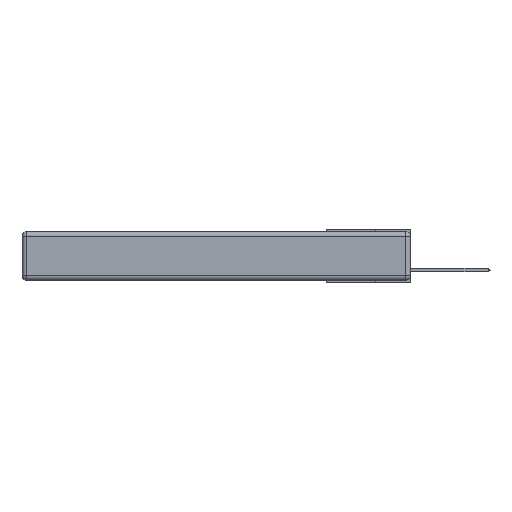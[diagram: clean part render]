
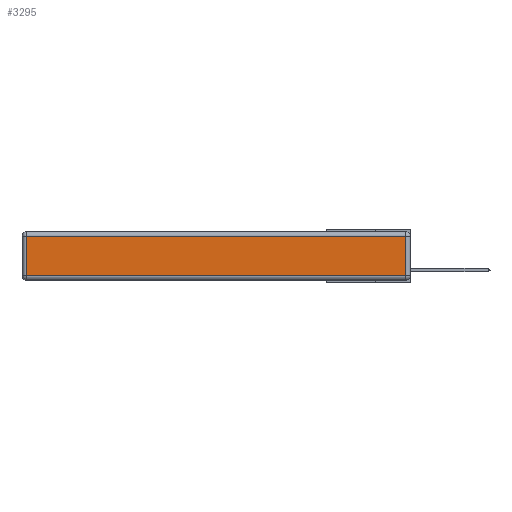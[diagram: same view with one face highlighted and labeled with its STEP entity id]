
A CAD part, left-side view. The second image highlights one B-rep face of the part: STEP entity #3295.
In plain terms, the highlighted planar face has unit normal (-1, 0, 0).
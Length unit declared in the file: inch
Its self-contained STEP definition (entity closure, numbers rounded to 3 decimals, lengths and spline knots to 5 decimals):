
#61 = CARTESIAN_POINT ( 'NONE',  ( 0., 0., -0.343 ) ) ;
#345 = EDGE_CURVE ( 'NONE', #7938, #7507, #6996, .T. ) ;
#945 = ORIENTED_EDGE ( 'NONE', *, *, #12163, .T. ) ;
#972 = EDGE_LOOP ( 'NONE', ( #12703, #6114, #8635, #945 ) ) ;
#1014 = CARTESIAN_POINT ( 'NONE',  ( 0., 0.03, -0.313 ) ) ;
#2079 = VECTOR ( 'NONE', #4748, 39.37008 ) ;
#2274 = EDGE_CURVE ( 'NONE', #4164, #7938, #5363, .T. ) ;
#3157 = DIRECTION ( 'NONE',  ( 0., -1., 0. ) ) ;
#3197 = VECTOR ( 'NONE', #7634, 39.37008 ) ;
#3209 = CARTESIAN_POINT ( 'NONE',  ( 0., 2.75, -0.03 ) ) ;
#3295 = ADVANCED_FACE ( 'NONE', ( #11266 ), #10130, .T. ) ;
#4022 = CARTESIAN_POINT ( 'NONE',  ( 0., 2.72, -0.03 ) ) ;
#4164 = VERTEX_POINT ( 'NONE', #1014 ) ;
#4319 = CARTESIAN_POINT ( 'NONE',  ( 0., 0., -0.313 ) ) ;
#4589 = DIRECTION ( 'NONE',  ( 0., 0., 1. ) ) ;
#4748 = DIRECTION ( 'NONE',  ( 0., 0., 1. ) ) ;
#4841 = LINE ( 'NONE', #4319, #8142 ) ;
#5363 = LINE ( 'NONE', #5771, #2079 ) ;
#5771 = CARTESIAN_POINT ( 'NONE',  ( 0., 0.03, -0.343 ) ) ;
#6088 = VERTEX_POINT ( 'NONE', #10136 ) ;
#6105 = DIRECTION ( 'NONE',  ( 0., 0., -1. ) ) ;
#6114 = ORIENTED_EDGE ( 'NONE', *, *, #2274, .T. ) ;
#6937 = AXIS2_PLACEMENT_3D ( 'NONE', #61, #13417, #4589 ) ;
#6996 = LINE ( 'NONE', #3209, #3197 ) ;
#7496 = LINE ( 'NONE', #13801, #13386 ) ;
#7507 = VERTEX_POINT ( 'NONE', #4022 ) ;
#7634 = DIRECTION ( 'NONE',  ( 0., 1., 0. ) ) ;
#7739 = CARTESIAN_POINT ( 'NONE',  ( 0., 0.03, -0.03 ) ) ;
#7938 = VERTEX_POINT ( 'NONE', #7739 ) ;
#8142 = VECTOR ( 'NONE', #3157, 39.37008 ) ;
#8635 = ORIENTED_EDGE ( 'NONE', *, *, #345, .T. ) ;
#10130 = PLANE ( 'NONE',  #6937 ) ;
#10136 = CARTESIAN_POINT ( 'NONE',  ( 0., 2.72, -0.313 ) ) ;
#10587 = EDGE_CURVE ( 'NONE', #6088, #4164, #4841, .T. ) ;
#11266 = FACE_OUTER_BOUND ( 'NONE', #972, .T. ) ;
#12163 = EDGE_CURVE ( 'NONE', #7507, #6088, #7496, .T. ) ;
#12703 = ORIENTED_EDGE ( 'NONE', *, *, #10587, .T. ) ;
#13386 = VECTOR ( 'NONE', #6105, 39.37008 ) ;
#13417 = DIRECTION ( 'NONE',  ( -1., 0., 0. ) ) ;
#13801 = CARTESIAN_POINT ( 'NONE',  ( 0., 2.72, -0.343 ) ) ;
